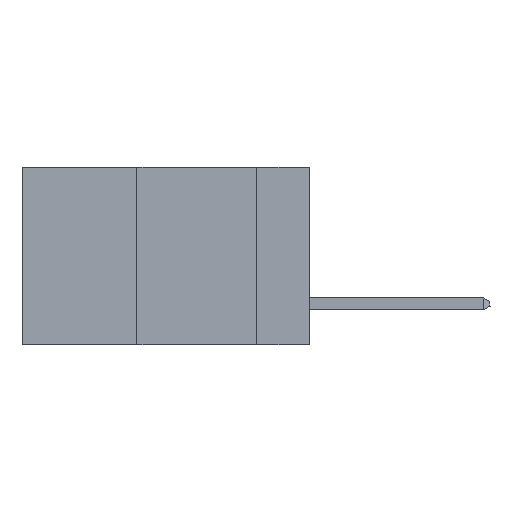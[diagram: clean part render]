
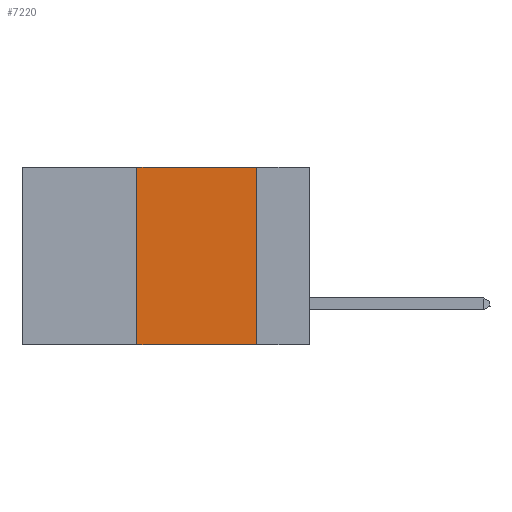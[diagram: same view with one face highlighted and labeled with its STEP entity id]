
A CAD part, left-side view. The second image highlights one B-rep face of the part: STEP entity #7220.
In plain terms, the highlighted planar face has unit normal (-1, 0, 0).
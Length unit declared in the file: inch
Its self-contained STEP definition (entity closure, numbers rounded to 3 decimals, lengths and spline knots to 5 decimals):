
#499 = EDGE_CURVE ( 'NONE', #12496, #6359, #9082, .T. ) ;
#502 = AXIS2_PLACEMENT_3D ( 'NONE', #1150, #4560, #6899 ) ;
#1043 = CARTESIAN_POINT ( 'NONE',  ( 0., 0.36, 0. ) ) ;
#1149 = CARTESIAN_POINT ( 'NONE',  ( 0., 0.6, 0. ) ) ;
#1150 = CARTESIAN_POINT ( 'NONE',  ( 0., 0.6, 0. ) ) ;
#1430 = CARTESIAN_POINT ( 'NONE',  ( 0., 0.11, 0. ) ) ;
#1523 = CARTESIAN_POINT ( 'NONE',  ( 0., 0.11, 0. ) ) ;
#1530 = PLANE ( 'NONE',  #502 ) ;
#1745 = CARTESIAN_POINT ( 'NONE',  ( 0., 0.36, -0.37 ) ) ;
#2306 = DIRECTION ( 'NONE',  ( 0., -1., 0. ) ) ;
#3210 = ORIENTED_EDGE ( 'NONE', *, *, #5981, .F. ) ;
#3315 = VECTOR ( 'NONE', #6494, 39.37008 ) ;
#3902 = CARTESIAN_POINT ( 'NONE',  ( 0., 0.6, -0.37 ) ) ;
#4560 = DIRECTION ( 'NONE',  ( 1., 0., 0. ) ) ;
#4684 = CARTESIAN_POINT ( 'NONE',  ( 0., 0.11, -0.37 ) ) ;
#4843 = VERTEX_POINT ( 'NONE', #8798 ) ;
#4870 = EDGE_CURVE ( 'NONE', #4843, #8877, #8272, .T. ) ;
#5256 = VECTOR ( 'NONE', #2306, 39.37008 ) ;
#5981 = EDGE_CURVE ( 'NONE', #12496, #4843, #10524, .T. ) ;
#6359 = VERTEX_POINT ( 'NONE', #4684 ) ;
#6494 = DIRECTION ( 'NONE',  ( 0., 0., 1. ) ) ;
#6899 = DIRECTION ( 'NONE',  ( 0., 0., -1. ) ) ;
#7143 = VECTOR ( 'NONE', #13854, 39.37008 ) ;
#7220 = ADVANCED_FACE ( 'NONE', ( #9688 ), #1530, .F. ) ;
#7349 = EDGE_LOOP ( 'NONE', ( #9284, #9216, #3210, #13548 ) ) ;
#8272 = LINE ( 'NONE', #1149, #5256 ) ;
#8798 = CARTESIAN_POINT ( 'NONE',  ( 0., 0.36, 0. ) ) ;
#8877 = VERTEX_POINT ( 'NONE', #1430 ) ;
#9082 = LINE ( 'NONE', #3902, #7143 ) ;
#9216 = ORIENTED_EDGE ( 'NONE', *, *, #4870, .F. ) ;
#9284 = ORIENTED_EDGE ( 'NONE', *, *, #11656, .F. ) ;
#9688 = FACE_OUTER_BOUND ( 'NONE', #7349, .T. ) ;
#10224 = LINE ( 'NONE', #1523, #11076 ) ;
#10524 = LINE ( 'NONE', #1043, #3315 ) ;
#11076 = VECTOR ( 'NONE', #12724, 39.37008 ) ;
#11656 = EDGE_CURVE ( 'NONE', #8877, #6359, #10224, .T. ) ;
#12496 = VERTEX_POINT ( 'NONE', #1745 ) ;
#12724 = DIRECTION ( 'NONE',  ( 0., 0., -1. ) ) ;
#13548 = ORIENTED_EDGE ( 'NONE', *, *, #499, .T. ) ;
#13854 = DIRECTION ( 'NONE',  ( 0., -1., 0. ) ) ;
